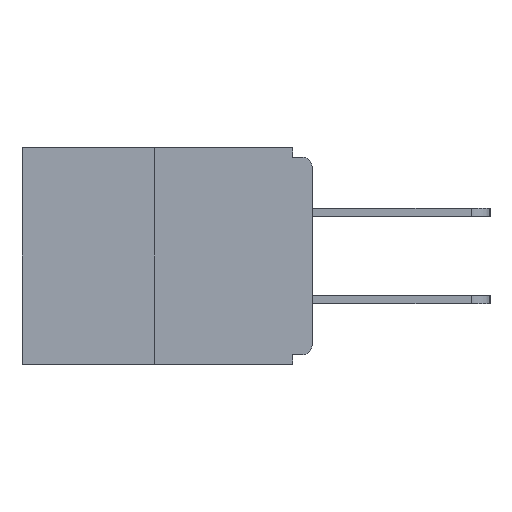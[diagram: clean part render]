
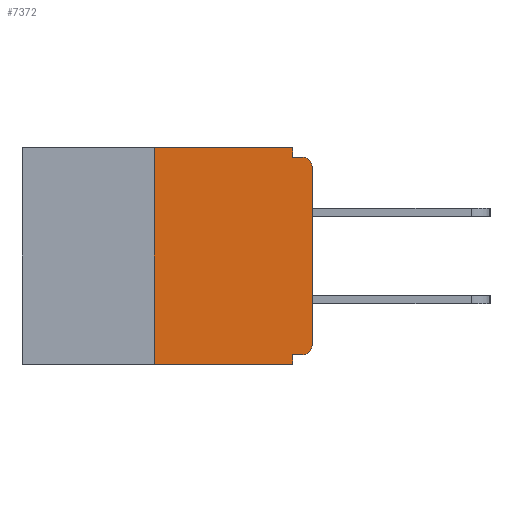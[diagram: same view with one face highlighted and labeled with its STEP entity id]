
A CAD part, left-side view. The second image highlights one B-rep face of the part: STEP entity #7372.
In plain terms, the highlighted planar face has unit normal (-1, 0, 0).
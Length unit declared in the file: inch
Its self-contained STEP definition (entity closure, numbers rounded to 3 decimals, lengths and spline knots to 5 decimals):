
#319 = ORIENTED_EDGE ( 'NONE', *, *, #12307, .T. ) ;
#382 = CARTESIAN_POINT ( 'NONE',  ( 0., 0.46, 0. ) ) ;
#599 = CARTESIAN_POINT ( 'NONE',  ( 0., 0.031, -0.328 ) ) ;
#637 = AXIS2_PLACEMENT_3D ( 'NONE', #13473, #828, #6460 ) ;
#806 = LINE ( 'NONE', #13457, #9839 ) ;
#828 = DIRECTION ( 'NONE',  ( -1., 0., 0. ) ) ;
#873 = ORIENTED_EDGE ( 'NONE', *, *, #13520, .F. ) ;
#976 = LINE ( 'NONE', #2763, #6044 ) ;
#1124 = LINE ( 'NONE', #4425, #6538 ) ;
#1285 = DIRECTION ( 'NONE',  ( 0., 0., -1. ) ) ;
#1286 = CARTESIAN_POINT ( 'NONE',  ( 0., 0.031, -0.015 ) ) ;
#1319 = EDGE_CURVE ( 'NONE', #14294, #8632, #1124, .T. ) ;
#1361 = LINE ( 'NONE', #9663, #14934 ) ;
#1398 = ORIENTED_EDGE ( 'NONE', *, *, #7655, .T. ) ;
#1580 = DIRECTION ( 'NONE',  ( 0., -1., 0. ) ) ;
#1829 = CARTESIAN_POINT ( 'NONE',  ( 0., 0.031, 0. ) ) ;
#1949 = VERTEX_POINT ( 'NONE', #12906 ) ;
#1954 = ORIENTED_EDGE ( 'NONE', *, *, #14542, .F. ) ;
#2140 = CIRCLE ( 'NONE', #637, 0.015 ) ;
#2592 = CARTESIAN_POINT ( 'NONE',  ( 0., 0.031, -0.343 ) ) ;
#2763 = CARTESIAN_POINT ( 'NONE',  ( 0., 0.46, 0. ) ) ;
#3205 = CARTESIAN_POINT ( 'NONE',  ( 0., 0., 0. ) ) ;
#4016 = FACE_OUTER_BOUND ( 'NONE', #4190, .T. ) ;
#4190 = EDGE_LOOP ( 'NONE', ( #873, #6193, #319, #1954, #9184, #1398, #6572, #8492, #11695, #10330 ) ) ;
#4425 = CARTESIAN_POINT ( 'NONE',  ( 0., 0.031, 0. ) ) ;
#4842 = CARTESIAN_POINT ( 'NONE',  ( 0., 0., -0.328 ) ) ;
#4935 = AXIS2_PLACEMENT_3D ( 'NONE', #9402, #12598, #10490 ) ;
#5346 = VERTEX_POINT ( 'NONE', #10685 ) ;
#5435 = EDGE_CURVE ( 'NONE', #5346, #9228, #13742, .T. ) ;
#5657 = CARTESIAN_POINT ( 'NONE',  ( 0., 0.25, 0. ) ) ;
#5684 = LINE ( 'NONE', #10371, #12343 ) ;
#5711 = CIRCLE ( 'NONE', #4935, 0.015 ) ;
#6044 = VECTOR ( 'NONE', #10374, 39.37008 ) ;
#6193 = ORIENTED_EDGE ( 'NONE', *, *, #10306, .F. ) ;
#6379 = VERTEX_POINT ( 'NONE', #10366 ) ;
#6460 = DIRECTION ( 'NONE',  ( 0., 0., -1. ) ) ;
#6538 = VECTOR ( 'NONE', #12772, 39.37008 ) ;
#6572 = ORIENTED_EDGE ( 'NONE', *, *, #14812, .T. ) ;
#6588 = DIRECTION ( 'NONE',  ( 0., 0., -1. ) ) ;
#7372 = ADVANCED_FACE ( 'NONE', ( #4016 ), #7730, .F. ) ;
#7433 = CARTESIAN_POINT ( 'NONE',  ( 0., 0., -0.015 ) ) ;
#7655 = EDGE_CURVE ( 'NONE', #5346, #1949, #5711, .T. ) ;
#7730 = PLANE ( 'NONE',  #9185 ) ;
#8492 = ORIENTED_EDGE ( 'NONE', *, *, #11060, .T. ) ;
#8632 = VERTEX_POINT ( 'NONE', #1286 ) ;
#8861 = VECTOR ( 'NONE', #1580, 39.37008 ) ;
#9124 = LINE ( 'NONE', #3205, #10222 ) ;
#9184 = ORIENTED_EDGE ( 'NONE', *, *, #5435, .F. ) ;
#9185 = AXIS2_PLACEMENT_3D ( 'NONE', #382, #12163, #6588 ) ;
#9228 = VERTEX_POINT ( 'NONE', #599 ) ;
#9402 = CARTESIAN_POINT ( 'NONE',  ( 0., 0.015, -0.313 ) ) ;
#9663 = CARTESIAN_POINT ( 'NONE',  ( 0., 0.031, -0.343 ) ) ;
#9700 = CARTESIAN_POINT ( 'NONE',  ( 0., 0.015, -0.015 ) ) ;
#9839 = VECTOR ( 'NONE', #14695, 39.37008 ) ;
#10146 = EDGE_CURVE ( 'NONE', #8632, #13264, #14377, .T. ) ;
#10222 = VECTOR ( 'NONE', #12619, 39.37008 ) ;
#10306 = EDGE_CURVE ( 'NONE', #6379, #13176, #806, .T. ) ;
#10330 = ORIENTED_EDGE ( 'NONE', *, *, #1319, .F. ) ;
#10366 = CARTESIAN_POINT ( 'NONE',  ( 0., 0.25, -0.343 ) ) ;
#10371 = CARTESIAN_POINT ( 'NONE',  ( 0., 0.46, -0.343 ) ) ;
#10374 = DIRECTION ( 'NONE',  ( 0., -1., 0. ) ) ;
#10490 = DIRECTION ( 'NONE',  ( 0., 0., -1. ) ) ;
#10685 = CARTESIAN_POINT ( 'NONE',  ( 0., 0.015, -0.328 ) ) ;
#10878 = VECTOR ( 'NONE', #12885, 39.37008 ) ;
#11060 = EDGE_CURVE ( 'NONE', #14563, #13264, #2140, .T. ) ;
#11368 = VERTEX_POINT ( 'NONE', #2592 ) ;
#11518 = DIRECTION ( 'NONE',  ( 0., -1., 0. ) ) ;
#11695 = ORIENTED_EDGE ( 'NONE', *, *, #10146, .F. ) ;
#11737 = CARTESIAN_POINT ( 'NONE',  ( 0., 0., -0.03 ) ) ;
#12163 = DIRECTION ( 'NONE',  ( 1., 0., 0. ) ) ;
#12307 = EDGE_CURVE ( 'NONE', #6379, #11368, #5684, .T. ) ;
#12343 = VECTOR ( 'NONE', #11518, 39.37008 ) ;
#12598 = DIRECTION ( 'NONE',  ( -1., 0., 0. ) ) ;
#12619 = DIRECTION ( 'NONE',  ( 0., 0., 1. ) ) ;
#12772 = DIRECTION ( 'NONE',  ( 0., 0., -1. ) ) ;
#12885 = DIRECTION ( 'NONE',  ( 0., 1., 0. ) ) ;
#12906 = CARTESIAN_POINT ( 'NONE',  ( 0., 0., -0.313 ) ) ;
#13176 = VERTEX_POINT ( 'NONE', #5657 ) ;
#13264 = VERTEX_POINT ( 'NONE', #9700 ) ;
#13457 = CARTESIAN_POINT ( 'NONE',  ( 0., 0.25, 0. ) ) ;
#13473 = CARTESIAN_POINT ( 'NONE',  ( 0., 0.015, -0.03 ) ) ;
#13520 = EDGE_CURVE ( 'NONE', #13176, #14294, #976, .T. ) ;
#13742 = LINE ( 'NONE', #4842, #10878 ) ;
#14294 = VERTEX_POINT ( 'NONE', #1829 ) ;
#14377 = LINE ( 'NONE', #7433, #8861 ) ;
#14542 = EDGE_CURVE ( 'NONE', #9228, #11368, #1361, .T. ) ;
#14563 = VERTEX_POINT ( 'NONE', #11737 ) ;
#14695 = DIRECTION ( 'NONE',  ( 0., 0., 1. ) ) ;
#14812 = EDGE_CURVE ( 'NONE', #1949, #14563, #9124, .T. ) ;
#14934 = VECTOR ( 'NONE', #1285, 39.37008 ) ;
